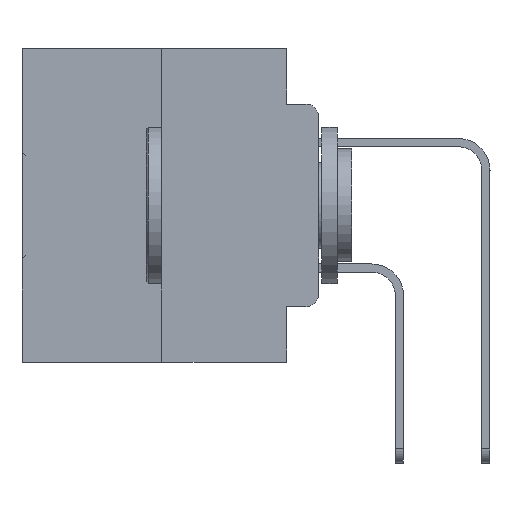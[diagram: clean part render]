
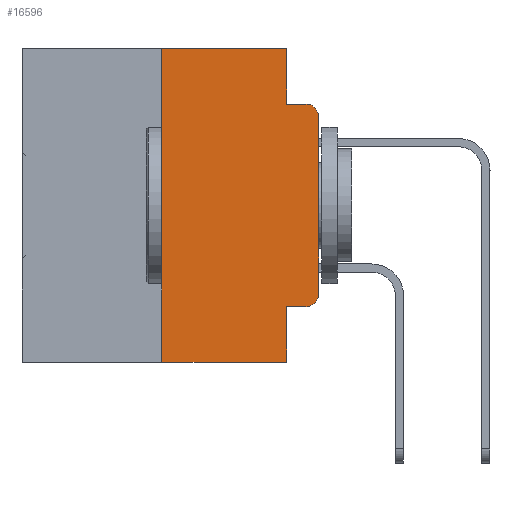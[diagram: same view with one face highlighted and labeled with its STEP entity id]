
A CAD part, left-side view. The second image highlights one B-rep face of the part: STEP entity #16596.
In plain terms, the highlighted planar face has unit normal (-1, 0, 0).
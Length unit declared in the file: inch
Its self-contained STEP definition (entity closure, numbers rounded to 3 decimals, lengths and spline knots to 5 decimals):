
#1465 = EDGE_CURVE ( 'NONE', #22105, #2674, #5877, .T. ) ;
#1852 = VERTEX_POINT ( 'NONE', #21993 ) ;
#1960 = ORIENTED_EDGE ( 'NONE', *, *, #1465, .T. ) ;
#2323 = LINE ( 'NONE', #5287, #23616 ) ;
#2674 = VERTEX_POINT ( 'NONE', #21209 ) ;
#2757 = CARTESIAN_POINT ( 'NONE',  ( 0., 0., -0.3915 ) ) ;
#3195 = ORIENTED_EDGE ( 'NONE', *, *, #23676, .T. ) ;
#3440 = VECTOR ( 'NONE', #9354, 39.37008 ) ;
#3643 = AXIS2_PLACEMENT_3D ( 'NONE', #26621, #29447, #21620 ) ;
#3705 = CARTESIAN_POINT ( 'NONE',  ( 0., 0.051, 0. ) ) ;
#3763 = VECTOR ( 'NONE', #9369, 39.37008 ) ;
#4686 = AXIS2_PLACEMENT_3D ( 'NONE', #5304, #13513, #24378 ) ;
#5287 = CARTESIAN_POINT ( 'NONE',  ( 0., 0.051, 0. ) ) ;
#5304 = CARTESIAN_POINT ( 'NONE',  ( 0., 0.473, 0. ) ) ;
#5646 = ORIENTED_EDGE ( 'NONE', *, *, #21483, .F. ) ;
#5877 = LINE ( 'NONE', #19607, #22970 ) ;
#6333 = ORIENTED_EDGE ( 'NONE', *, *, #26786, .T. ) ;
#7802 = CARTESIAN_POINT ( 'NONE',  ( 0., 0.473, -0.5 ) ) ;
#8337 = ORIENTED_EDGE ( 'NONE', *, *, #18966, .T. ) ;
#9354 = DIRECTION ( 'NONE',  ( 0., -1., 0. ) ) ;
#9369 = DIRECTION ( 'NONE',  ( 0., 0., 1. ) ) ;
#9625 = VECTOR ( 'NONE', #24526, 39.37008 ) ;
#9899 = ORIENTED_EDGE ( 'NONE', *, *, #14696, .F. ) ;
#10364 = DIRECTION ( 'NONE',  ( 0., -1., 0. ) ) ;
#10985 = LINE ( 'NONE', #20139, #3763 ) ;
#12070 = VECTOR ( 'NONE', #10364, 39.37008 ) ;
#12193 = ORIENTED_EDGE ( 'NONE', *, *, #23980, .F. ) ;
#12239 = CARTESIAN_POINT ( 'NONE',  ( 0., 0.051, -0.0885 ) ) ;
#12396 = LINE ( 'NONE', #12239, #3440 ) ;
#12623 = VERTEX_POINT ( 'NONE', #2757 ) ;
#13053 = VERTEX_POINT ( 'NONE', #29183 ) ;
#13513 = DIRECTION ( 'NONE',  ( 1., 0., 0. ) ) ;
#14198 = VERTEX_POINT ( 'NONE', #23393 ) ;
#14696 = EDGE_CURVE ( 'NONE', #20072, #17200, #10985, .T. ) ;
#16253 = LINE ( 'NONE', #17933, #28195 ) ;
#16596 = ADVANCED_FACE ( 'NONE', ( #23476 ), #18769, .F. ) ;
#17200 = VERTEX_POINT ( 'NONE', #21487 ) ;
#17933 = CARTESIAN_POINT ( 'NONE',  ( 0., 0.051, 0. ) ) ;
#18769 = PLANE ( 'NONE',  #4686 ) ;
#18838 = CARTESIAN_POINT ( 'NONE',  ( 0., 0.02, -0.3915 ) ) ;
#18966 = EDGE_CURVE ( 'NONE', #20072, #1852, #27580, .T. ) ;
#19073 = DIRECTION ( 'NONE',  ( -1., 0., 0. ) ) ;
#19103 = DIRECTION ( 'NONE',  ( 0., 0., -1. ) ) ;
#19607 = CARTESIAN_POINT ( 'NONE',  ( 0., 0.051, -0.4115 ) ) ;
#20072 = VERTEX_POINT ( 'NONE', #28695 ) ;
#20139 = CARTESIAN_POINT ( 'NONE',  ( 0., 0.25, 0. ) ) ;
#20691 = DIRECTION ( 'NONE',  ( 0., 0., 1. ) ) ;
#20954 = EDGE_CURVE ( 'NONE', #13053, #14198, #21865, .T. ) ;
#20997 = CARTESIAN_POINT ( 'NONE',  ( 0., 0.051, -0.4115 ) ) ;
#21209 = CARTESIAN_POINT ( 'NONE',  ( 0., 0.02, -0.4115 ) ) ;
#21483 = EDGE_CURVE ( 'NONE', #22105, #1852, #16253, .T. ) ;
#21487 = CARTESIAN_POINT ( 'NONE',  ( 0., 0.25, 0. ) ) ;
#21620 = DIRECTION ( 'NONE',  ( 0., 0., -1. ) ) ;
#21865 = CIRCLE ( 'NONE', #3643, 0.02 ) ;
#21993 = CARTESIAN_POINT ( 'NONE',  ( 0., 0.051, -0.5 ) ) ;
#22105 = VERTEX_POINT ( 'NONE', #20997 ) ;
#22970 = VECTOR ( 'NONE', #27487, 39.37008 ) ;
#23058 = ORIENTED_EDGE ( 'NONE', *, *, #28398, .F. ) ;
#23393 = CARTESIAN_POINT ( 'NONE',  ( 0., 0.02, -0.0885 ) ) ;
#23476 = FACE_OUTER_BOUND ( 'NONE', #28749, .T. ) ;
#23616 = VECTOR ( 'NONE', #19103, 39.37008 ) ;
#23676 = EDGE_CURVE ( 'NONE', #2674, #12623, #32476, .T. ) ;
#23980 = EDGE_CURVE ( 'NONE', #28630, #14198, #12396, .T. ) ;
#24378 = DIRECTION ( 'NONE',  ( 0., 0., -1. ) ) ;
#24526 = DIRECTION ( 'NONE',  ( 0., -1., 0. ) ) ;
#25460 = VECTOR ( 'NONE', #20691, 39.37008 ) ;
#26621 = CARTESIAN_POINT ( 'NONE',  ( 0., 0.02, -0.1085 ) ) ;
#26786 = EDGE_CURVE ( 'NONE', #12623, #13053, #30986, .T. ) ;
#27487 = DIRECTION ( 'NONE',  ( 0., -1., 0. ) ) ;
#27580 = LINE ( 'NONE', #7802, #9625 ) ;
#28195 = VECTOR ( 'NONE', #28794, 39.37008 ) ;
#28398 = EDGE_CURVE ( 'NONE', #28661, #28630, #2323, .T. ) ;
#28630 = VERTEX_POINT ( 'NONE', #31251 ) ;
#28661 = VERTEX_POINT ( 'NONE', #3705 ) ;
#28695 = CARTESIAN_POINT ( 'NONE',  ( 0., 0.25, -0.5 ) ) ;
#28749 = EDGE_LOOP ( 'NONE', ( #6333, #29731, #12193, #23058, #29254, #9899, #8337, #5646, #1960, #3195 ) ) ;
#28794 = DIRECTION ( 'NONE',  ( 0., 0., -1. ) ) ;
#29183 = CARTESIAN_POINT ( 'NONE',  ( 0., 0., -0.1085 ) ) ;
#29254 = ORIENTED_EDGE ( 'NONE', *, *, #29334, .F. ) ;
#29334 = EDGE_CURVE ( 'NONE', #17200, #28661, #34696, .T. ) ;
#29447 = DIRECTION ( 'NONE',  ( -1., 0., 0. ) ) ;
#29731 = ORIENTED_EDGE ( 'NONE', *, *, #20954, .T. ) ;
#29901 = DIRECTION ( 'NONE',  ( 0., 0., -1. ) ) ;
#30986 = LINE ( 'NONE', #31176, #25460 ) ;
#31176 = CARTESIAN_POINT ( 'NONE',  ( 0., 0., 0. ) ) ;
#31251 = CARTESIAN_POINT ( 'NONE',  ( 0., 0.051, -0.0885 ) ) ;
#32476 = CIRCLE ( 'NONE', #34058, 0.02 ) ;
#34058 = AXIS2_PLACEMENT_3D ( 'NONE', #18838, #19073, #29901 ) ;
#34696 = LINE ( 'NONE', #35274, #12070 ) ;
#35274 = CARTESIAN_POINT ( 'NONE',  ( 0., 0.473, 0. ) ) ;
